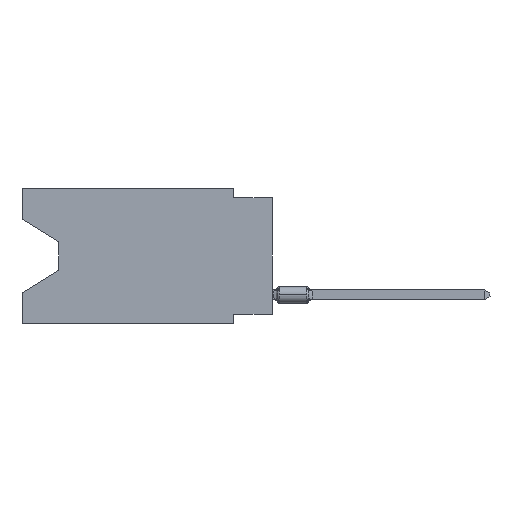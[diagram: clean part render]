
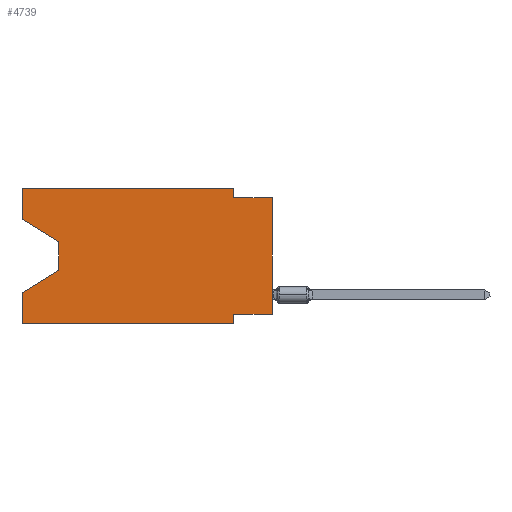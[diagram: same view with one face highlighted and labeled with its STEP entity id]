
A CAD part, left-side view. The second image highlights one B-rep face of the part: STEP entity #4739.
In plain terms, the highlighted planar face has unit normal (-1, 0, 0).
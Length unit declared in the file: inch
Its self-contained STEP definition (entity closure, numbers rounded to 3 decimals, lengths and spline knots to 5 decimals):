
#17 = CARTESIAN_POINT ( 'NONE',  ( 0., 0.645, -0.08025 ) ) ;
#57 = ORIENTED_EDGE ( 'NONE', *, *, #4833, .F. ) ;
#308 = VECTOR ( 'NONE', #7842, 39.37008 ) ;
#337 = LINE ( 'NONE', #10544, #308 ) ;
#596 = LINE ( 'NONE', #23341, #22603 ) ;
#1054 = VECTOR ( 'NONE', #24177, 39.37008 ) ;
#1298 = EDGE_CURVE ( 'NONE', #8252, #14805, #337, .T. ) ;
#1533 = ORIENTED_EDGE ( 'NONE', *, *, #4186, .F. ) ;
#1863 = VERTEX_POINT ( 'NONE', #12961 ) ;
#1998 = CARTESIAN_POINT ( 'NONE',  ( 0., 0.1, 0. ) ) ;
#3514 = LINE ( 'NONE', #11040, #1054 ) ;
#3750 = DIRECTION ( 'NONE',  ( 0., 0., -1. ) ) ;
#3813 = VECTOR ( 'NONE', #17207, 39.37008 ) ;
#4099 = DIRECTION ( 'NONE',  ( 0., 0., -1. ) ) ;
#4105 = EDGE_CURVE ( 'NONE', #16593, #16902, #9707, .T. ) ;
#4186 = EDGE_CURVE ( 'NONE', #16593, #14066, #5118, .T. ) ;
#4242 = CARTESIAN_POINT ( 'NONE',  ( 0., 0.645, -0.35 ) ) ;
#4351 = EDGE_CURVE ( 'NONE', #6237, #23162, #3514, .T. ) ;
#4739 = ADVANCED_FACE ( 'NONE', ( #5346 ), #12866, .F. ) ;
#4824 = ORIENTED_EDGE ( 'NONE', *, *, #18845, .F. ) ;
#4833 = EDGE_CURVE ( 'NONE', #1863, #19039, #22541, .T. ) ;
#5118 = LINE ( 'NONE', #21610, #12487 ) ;
#5132 = CARTESIAN_POINT ( 'NONE',  ( 0., 0., -0.025 ) ) ;
#5346 = FACE_OUTER_BOUND ( 'NONE', #10802, .T. ) ;
#5911 = CARTESIAN_POINT ( 'NONE',  ( 0., 0.645, -0.26975 ) ) ;
#5926 = DIRECTION ( 'NONE',  ( 0., -1., 0. ) ) ;
#6151 = LINE ( 'NONE', #13308, #10671 ) ;
#6237 = VERTEX_POINT ( 'NONE', #7774 ) ;
#6887 = CARTESIAN_POINT ( 'NONE',  ( 0., 0.1, -0.025 ) ) ;
#7172 = ORIENTED_EDGE ( 'NONE', *, *, #16544, .F. ) ;
#7490 = LINE ( 'NONE', #9347, #7543 ) ;
#7543 = VECTOR ( 'NONE', #22868, 39.37008 ) ;
#7571 = VECTOR ( 'NONE', #4099, 39.37008 ) ;
#7584 = ORIENTED_EDGE ( 'NONE', *, *, #20897, .F. ) ;
#7774 = CARTESIAN_POINT ( 'NONE',  ( 0., 0.55, -0.138 ) ) ;
#7794 = EDGE_CURVE ( 'NONE', #19039, #14805, #7490, .T. ) ;
#7842 = DIRECTION ( 'NONE',  ( 0., 0., 1. ) ) ;
#8252 = VERTEX_POINT ( 'NONE', #17457 ) ;
#8500 = VECTOR ( 'NONE', #20738, 39.37008 ) ;
#8615 = CARTESIAN_POINT ( 'NONE',  ( 0., 0.645, 0. ) ) ;
#9253 = LINE ( 'NONE', #17, #15494 ) ;
#9260 = DIRECTION ( 'NONE',  ( 1., 0., 0. ) ) ;
#9273 = LINE ( 'NONE', #20608, #22055 ) ;
#9347 = CARTESIAN_POINT ( 'NONE',  ( 0., 0., -0.025 ) ) ;
#9683 = LINE ( 'NONE', #20989, #8500 ) ;
#9707 = LINE ( 'NONE', #17320, #3813 ) ;
#10544 = CARTESIAN_POINT ( 'NONE',  ( 0., 0., 0. ) ) ;
#10671 = VECTOR ( 'NONE', #13676, 39.37008 ) ;
#10802 = EDGE_LOOP ( 'NONE', ( #22770, #19625, #18428, #1533, #23856, #7172, #7584, #23036, #20275, #57, #20594, #4824 ) ) ;
#11040 = CARTESIAN_POINT ( 'NONE',  ( 0., 0.55, -0.138 ) ) ;
#11451 = CARTESIAN_POINT ( 'NONE',  ( 0., 0.645, -0.08025 ) ) ;
#12487 = VECTOR ( 'NONE', #14242, 39.37008 ) ;
#12866 = PLANE ( 'NONE',  #19549 ) ;
#12961 = CARTESIAN_POINT ( 'NONE',  ( 0., 0.1, 0. ) ) ;
#13308 = CARTESIAN_POINT ( 'NONE',  ( 0., 0.645, 0. ) ) ;
#13519 = CARTESIAN_POINT ( 'NONE',  ( 0., 0.55, -0.212 ) ) ;
#13676 = DIRECTION ( 'NONE',  ( 0., 0., 1. ) ) ;
#14066 = VERTEX_POINT ( 'NONE', #5911 ) ;
#14242 = DIRECTION ( 'NONE',  ( 0., 0., 1. ) ) ;
#14477 = VERTEX_POINT ( 'NONE', #8615 ) ;
#14734 = EDGE_CURVE ( 'NONE', #23162, #14066, #596, .T. ) ;
#14805 = VERTEX_POINT ( 'NONE', #5132 ) ;
#14926 = DIRECTION ( 'NONE',  ( 0., 0., -1. ) ) ;
#15292 = LINE ( 'NONE', #17631, #20986 ) ;
#15494 = VECTOR ( 'NONE', #20817, 39.37008 ) ;
#15500 = DIRECTION ( 'NONE',  ( 0., 0.855, -0.519 ) ) ;
#16544 = EDGE_CURVE ( 'NONE', #24287, #16902, #9273, .T. ) ;
#16593 = VERTEX_POINT ( 'NONE', #4242 ) ;
#16719 = CARTESIAN_POINT ( 'NONE',  ( 0., 0.1, -0.325 ) ) ;
#16902 = VERTEX_POINT ( 'NONE', #22371 ) ;
#17207 = DIRECTION ( 'NONE',  ( 0., -1., 0. ) ) ;
#17320 = CARTESIAN_POINT ( 'NONE',  ( 0., 0.645, -0.35 ) ) ;
#17457 = CARTESIAN_POINT ( 'NONE',  ( 0., 0., -0.325 ) ) ;
#17631 = CARTESIAN_POINT ( 'NONE',  ( 0., 0.645, 0. ) ) ;
#17650 = VERTEX_POINT ( 'NONE', #11451 ) ;
#18277 = CARTESIAN_POINT ( 'NONE',  ( 0., 0.645, 0. ) ) ;
#18428 = ORIENTED_EDGE ( 'NONE', *, *, #14734, .T. ) ;
#18845 = EDGE_CURVE ( 'NONE', #17650, #14477, #6151, .T. ) ;
#19039 = VERTEX_POINT ( 'NONE', #6887 ) ;
#19549 = AXIS2_PLACEMENT_3D ( 'NONE', #18277, #9260, #14926 ) ;
#19625 = ORIENTED_EDGE ( 'NONE', *, *, #4351, .T. ) ;
#20275 = ORIENTED_EDGE ( 'NONE', *, *, #7794, .F. ) ;
#20594 = ORIENTED_EDGE ( 'NONE', *, *, #23488, .F. ) ;
#20608 = CARTESIAN_POINT ( 'NONE',  ( 0., 0.1, -0.35 ) ) ;
#20738 = DIRECTION ( 'NONE',  ( 0., 1., 0. ) ) ;
#20817 = DIRECTION ( 'NONE',  ( 0., -0.855, -0.519 ) ) ;
#20897 = EDGE_CURVE ( 'NONE', #8252, #24287, #9683, .T. ) ;
#20986 = VECTOR ( 'NONE', #5926, 39.37008 ) ;
#20989 = CARTESIAN_POINT ( 'NONE',  ( 0., 0., -0.325 ) ) ;
#21610 = CARTESIAN_POINT ( 'NONE',  ( 0., 0.645, 0. ) ) ;
#22055 = VECTOR ( 'NONE', #3750, 39.37008 ) ;
#22371 = CARTESIAN_POINT ( 'NONE',  ( 0., 0.1, -0.35 ) ) ;
#22541 = LINE ( 'NONE', #1998, #7571 ) ;
#22603 = VECTOR ( 'NONE', #15500, 39.37008 ) ;
#22770 = ORIENTED_EDGE ( 'NONE', *, *, #23369, .T. ) ;
#22868 = DIRECTION ( 'NONE',  ( 0., -1., 0. ) ) ;
#23036 = ORIENTED_EDGE ( 'NONE', *, *, #1298, .T. ) ;
#23162 = VERTEX_POINT ( 'NONE', #13519 ) ;
#23341 = CARTESIAN_POINT ( 'NONE',  ( 0., 0.55, -0.212 ) ) ;
#23369 = EDGE_CURVE ( 'NONE', #17650, #6237, #9253, .T. ) ;
#23488 = EDGE_CURVE ( 'NONE', #14477, #1863, #15292, .T. ) ;
#23856 = ORIENTED_EDGE ( 'NONE', *, *, #4105, .T. ) ;
#24177 = DIRECTION ( 'NONE',  ( 0., 0., -1. ) ) ;
#24287 = VERTEX_POINT ( 'NONE', #16719 ) ;
